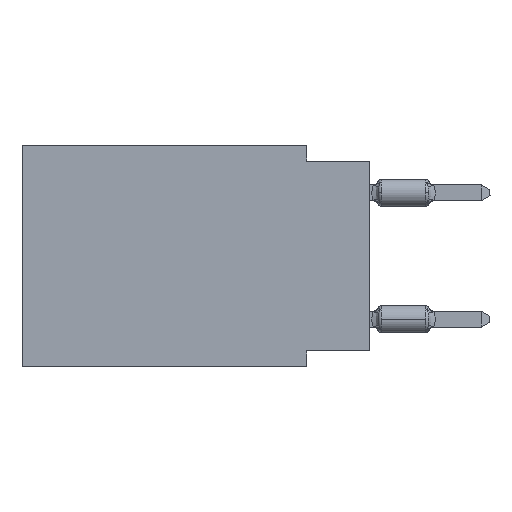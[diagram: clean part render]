
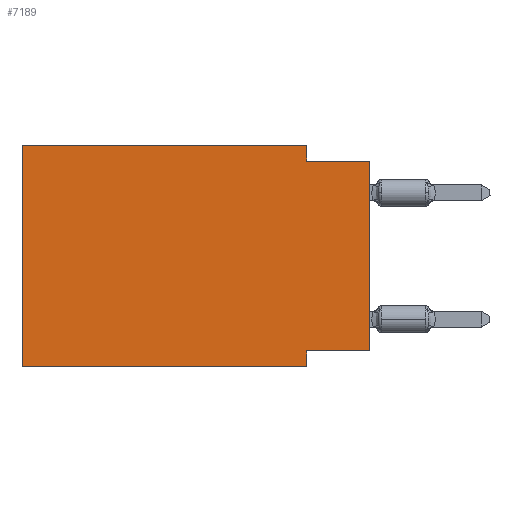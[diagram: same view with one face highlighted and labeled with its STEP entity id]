
A CAD part, left-side view. The second image highlights one B-rep face of the part: STEP entity #7189.
In plain terms, the highlighted planar face has unit normal (-1, 0, 0).
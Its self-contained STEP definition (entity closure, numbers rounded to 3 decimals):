
#20 = ORIENTED_EDGE ( 'NONE', *, *, #13119, .F. ) ;
#1564 = ORIENTED_EDGE ( 'NONE', *, *, #14106, .F. ) ;
#1812 = DIRECTION ( 'NONE',  ( 0., 0., 1. ) ) ;
#2845 = LINE ( 'NONE', #13693, #18302 ) ;
#4373 = CARTESIAN_POINT ( 'NONE',  ( 0., 2.54, -8.89 ) ) ;
#5426 = LINE ( 'NONE', #18875, #13386 ) ;
#6009 = CARTESIAN_POINT ( 'NONE',  ( 0., 2.54, 0. ) ) ;
#6473 = AXIS2_PLACEMENT_3D ( 'NONE', #28462, #8299, #28036 ) ;
#6538 = VECTOR ( 'NONE', #42511, 1000. ) ;
#6946 = VERTEX_POINT ( 'NONE', #26548 ) ;
#7167 = LINE ( 'NONE', #16078, #6538 ) ;
#7189 = ADVANCED_FACE ( 'NONE', ( #41030 ), #41254, .F. ) ;
#7352 = VECTOR ( 'NONE', #1812, 1000. ) ;
#7540 = EDGE_LOOP ( 'NONE', ( #14383, #20, #42001, #1564, #35828, #26954, #7694, #41613 ) ) ;
#7694 = ORIENTED_EDGE ( 'NONE', *, *, #19091, .F. ) ;
#7708 = VECTOR ( 'NONE', #8616, 1000. ) ;
#8289 = EDGE_CURVE ( 'NONE', #15429, #15907, #19903, .T. ) ;
#8299 = DIRECTION ( 'NONE',  ( 1., 0., 0. ) ) ;
#8616 = DIRECTION ( 'NONE',  ( 0., 0., -1. ) ) ;
#10068 = EDGE_CURVE ( 'NONE', #42792, #37027, #25635, .T. ) ;
#10880 = VECTOR ( 'NONE', #33110, 1000. ) ;
#12454 = VERTEX_POINT ( 'NONE', #14842 ) ;
#13119 = EDGE_CURVE ( 'NONE', #15907, #6946, #2845, .T. ) ;
#13167 = EDGE_CURVE ( 'NONE', #12454, #41436, #7167, .T. ) ;
#13386 = VECTOR ( 'NONE', #32080, 1000. ) ;
#13693 = CARTESIAN_POINT ( 'NONE',  ( 0., 0., -0.635 ) ) ;
#14106 = EDGE_CURVE ( 'NONE', #37027, #15429, #38949, .T. ) ;
#14383 = ORIENTED_EDGE ( 'NONE', *, *, #33569, .T. ) ;
#14842 = CARTESIAN_POINT ( 'NONE',  ( 0., 0., -8.255 ) ) ;
#15429 = VERTEX_POINT ( 'NONE', #6009 ) ;
#15907 = VERTEX_POINT ( 'NONE', #29362 ) ;
#16078 = CARTESIAN_POINT ( 'NONE',  ( 0., 0., -8.255 ) ) ;
#16297 = DIRECTION ( 'NONE',  ( 0., -1., 0. ) ) ;
#18286 = CARTESIAN_POINT ( 'NONE',  ( 0., 13.97, 0. ) ) ;
#18302 = VECTOR ( 'NONE', #16297, 1000. ) ;
#18875 = CARTESIAN_POINT ( 'NONE',  ( 0., 0., 0. ) ) ;
#19091 = EDGE_CURVE ( 'NONE', #41436, #32693, #19430, .T. ) ;
#19430 = LINE ( 'NONE', #38298, #7708 ) ;
#19903 = LINE ( 'NONE', #27036, #10880 ) ;
#22236 = CARTESIAN_POINT ( 'NONE',  ( 0., 13.97, 0. ) ) ;
#25635 = LINE ( 'NONE', #18286, #7352 ) ;
#26223 = EDGE_CURVE ( 'NONE', #42792, #32693, #36664, .T. ) ;
#26548 = CARTESIAN_POINT ( 'NONE',  ( 0., 0., -0.635 ) ) ;
#26954 = ORIENTED_EDGE ( 'NONE', *, *, #26223, .T. ) ;
#27036 = CARTESIAN_POINT ( 'NONE',  ( 0., 2.54, 0. ) ) ;
#28014 = VECTOR ( 'NONE', #35229, 1000. ) ;
#28036 = DIRECTION ( 'NONE',  ( 0., 0., -1. ) ) ;
#28462 = CARTESIAN_POINT ( 'NONE',  ( 0., 13.97, 0. ) ) ;
#29362 = CARTESIAN_POINT ( 'NONE',  ( 0., 2.54, -0.635 ) ) ;
#30181 = CARTESIAN_POINT ( 'NONE',  ( 0., 13.97, -8.89 ) ) ;
#32080 = DIRECTION ( 'NONE',  ( 0., 0., 1. ) ) ;
#32693 = VERTEX_POINT ( 'NONE', #4373 ) ;
#33110 = DIRECTION ( 'NONE',  ( 0., 0., -1. ) ) ;
#33569 = EDGE_CURVE ( 'NONE', #12454, #6946, #5426, .T. ) ;
#35229 = DIRECTION ( 'NONE',  ( 0., -1., 0. ) ) ;
#35482 = DIRECTION ( 'NONE',  ( 0., -1., 0. ) ) ;
#35828 = ORIENTED_EDGE ( 'NONE', *, *, #10068, .F. ) ;
#36664 = LINE ( 'NONE', #30181, #28014 ) ;
#37027 = VERTEX_POINT ( 'NONE', #22236 ) ;
#38298 = CARTESIAN_POINT ( 'NONE',  ( 0., 2.54, -8.89 ) ) ;
#38531 = CARTESIAN_POINT ( 'NONE',  ( 0., 13.97, 0. ) ) ;
#38949 = LINE ( 'NONE', #38531, #40501 ) ;
#39155 = CARTESIAN_POINT ( 'NONE',  ( 0., 13.97, -8.89 ) ) ;
#40501 = VECTOR ( 'NONE', #35482, 1000. ) ;
#41030 = FACE_OUTER_BOUND ( 'NONE', #7540, .T. ) ;
#41110 = CARTESIAN_POINT ( 'NONE',  ( 0., 2.54, -8.255 ) ) ;
#41254 = PLANE ( 'NONE',  #6473 ) ;
#41436 = VERTEX_POINT ( 'NONE', #41110 ) ;
#41613 = ORIENTED_EDGE ( 'NONE', *, *, #13167, .F. ) ;
#42001 = ORIENTED_EDGE ( 'NONE', *, *, #8289, .F. ) ;
#42511 = DIRECTION ( 'NONE',  ( 0., 1., 0. ) ) ;
#42792 = VERTEX_POINT ( 'NONE', #39155 ) ;
